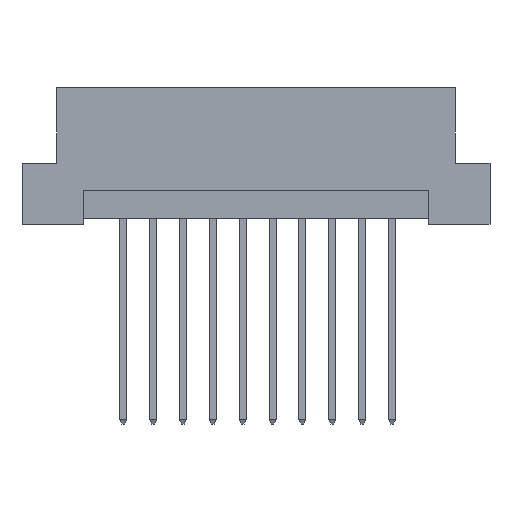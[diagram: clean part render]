
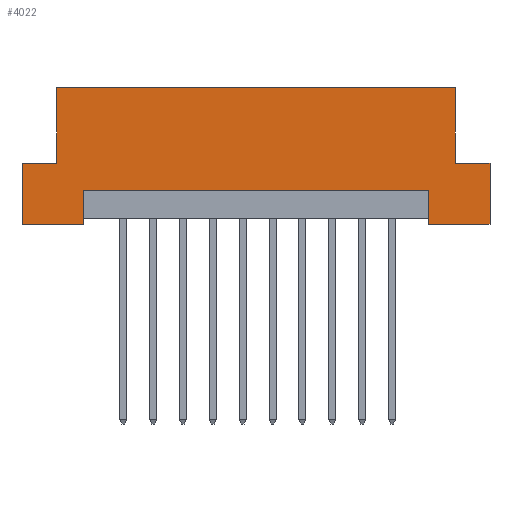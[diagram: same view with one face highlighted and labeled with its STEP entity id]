
A CAD part, front view. The second image highlights one B-rep face of the part: STEP entity #4022.
In plain terms, the highlighted planar face has unit normal (0, -1, 0).
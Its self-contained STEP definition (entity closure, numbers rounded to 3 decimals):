
#50 = CARTESIAN_POINT ( 'NONE',  ( 19.9, 0., 5.2 ) ) ;
#262 = EDGE_LOOP ( 'NONE', ( #6584, #5447, #4503, #2986, #5930, #6435, #2217, #4300, #5325, #4414, #3170, #342 ) ) ;
#336 = LINE ( 'NONE', #4643, #783 ) ;
#342 = ORIENTED_EDGE ( 'NONE', *, *, #4742, .F. ) ;
#356 = PLANE ( 'NONE',  #2508 ) ;
#554 = CARTESIAN_POINT ( 'NONE',  ( -19.9, 0., 5.2 ) ) ;
#592 = CARTESIAN_POINT ( 'NONE',  ( -19.9, 0., 5.2 ) ) ;
#783 = VECTOR ( 'NONE', #5684, 1000. ) ;
#797 = EDGE_CURVE ( 'NONE', #2277, #6769, #2250, .T. ) ;
#870 = CARTESIAN_POINT ( 'NONE',  ( 19.9, 0., 0. ) ) ;
#879 = VECTOR ( 'NONE', #4451, 1000. ) ;
#881 = CARTESIAN_POINT ( 'NONE',  ( -19.9, 0., 0. ) ) ;
#1060 = VECTOR ( 'NONE', #2801, 1000. ) ;
#1104 = EDGE_CURVE ( 'NONE', #5030, #2450, #3329, .T. ) ;
#1120 = LINE ( 'NONE', #592, #4772 ) ;
#1385 = LINE ( 'NONE', #6253, #3183 ) ;
#1445 = CARTESIAN_POINT ( 'NONE',  ( -19.9, 0., 11.6 ) ) ;
#1475 = EDGE_CURVE ( 'NONE', #1818, #4754, #336, .T. ) ;
#1507 = DIRECTION ( 'NONE',  ( 0., 0., 1. ) ) ;
#1660 = LINE ( 'NONE', #5497, #1060 ) ;
#1763 = VERTEX_POINT ( 'NONE', #6901 ) ;
#1818 = VERTEX_POINT ( 'NONE', #3364 ) ;
#1860 = VECTOR ( 'NONE', #6773, 1000. ) ;
#1890 = CARTESIAN_POINT ( 'NONE',  ( -19.9, 0., 0. ) ) ;
#1901 = CARTESIAN_POINT ( 'NONE',  ( -14.69, 0., 0.5 ) ) ;
#2171 = VERTEX_POINT ( 'NONE', #6325 ) ;
#2204 = DIRECTION ( 'NONE',  ( 1., 0., 0. ) ) ;
#2215 = CARTESIAN_POINT ( 'NONE',  ( 14.69, 0., 2.9 ) ) ;
#2217 = ORIENTED_EDGE ( 'NONE', *, *, #1475, .F. ) ;
#2250 = LINE ( 'NONE', #2215, #2349 ) ;
#2277 = VERTEX_POINT ( 'NONE', #3214 ) ;
#2349 = VECTOR ( 'NONE', #5944, 1000. ) ;
#2450 = VERTEX_POINT ( 'NONE', #2934 ) ;
#2483 = EDGE_CURVE ( 'NONE', #2450, #6653, #4736, .T. ) ;
#2508 = AXIS2_PLACEMENT_3D ( 'NONE', #1445, #6988, #1507 ) ;
#2801 = DIRECTION ( 'NONE',  ( 0., 0., 1. ) ) ;
#2822 = EDGE_CURVE ( 'NONE', #2171, #1818, #5633, .T. ) ;
#2891 = LINE ( 'NONE', #1901, #1860 ) ;
#2904 = LINE ( 'NONE', #3502, #5082 ) ;
#2934 = CARTESIAN_POINT ( 'NONE',  ( 19.9, 0., 5.2 ) ) ;
#2986 = ORIENTED_EDGE ( 'NONE', *, *, #2483, .F. ) ;
#3008 = LINE ( 'NONE', #881, #6838 ) ;
#3039 = DIRECTION ( 'NONE',  ( -1., 0., 0. ) ) ;
#3167 = DIRECTION ( 'NONE',  ( 0., 0., -1. ) ) ;
#3170 = ORIENTED_EDGE ( 'NONE', *, *, #3307, .F. ) ;
#3175 = CARTESIAN_POINT ( 'NONE',  ( -14.69, 0., 2.9 ) ) ;
#3183 = VECTOR ( 'NONE', #5683, 1000. ) ;
#3214 = CARTESIAN_POINT ( 'NONE',  ( 14.69, 0., 2.9 ) ) ;
#3263 = VERTEX_POINT ( 'NONE', #1890 ) ;
#3307 = EDGE_CURVE ( 'NONE', #4522, #3263, #1385, .T. ) ;
#3326 = EDGE_CURVE ( 'NONE', #6653, #1763, #3008, .T. ) ;
#3329 = LINE ( 'NONE', #50, #5870 ) ;
#3364 = CARTESIAN_POINT ( 'NONE',  ( -16.94, 0., 11.6 ) ) ;
#3483 = VECTOR ( 'NONE', #3167, 1000. ) ;
#3502 = CARTESIAN_POINT ( 'NONE',  ( 16.94, 0., 5.2 ) ) ;
#3712 = EDGE_CURVE ( 'NONE', #3263, #4529, #1660, .T. ) ;
#3883 = LINE ( 'NONE', #5023, #5916 ) ;
#3956 = DIRECTION ( 'NONE',  ( 0., 0., 1. ) ) ;
#4022 = ADVANCED_FACE ( 'NONE', ( #5272 ), #356, .F. ) ;
#4300 = ORIENTED_EDGE ( 'NONE', *, *, #2822, .F. ) ;
#4414 = ORIENTED_EDGE ( 'NONE', *, *, #3712, .F. ) ;
#4442 = CARTESIAN_POINT ( 'NONE',  ( 16.94, 0., 11.6 ) ) ;
#4451 = DIRECTION ( 'NONE',  ( 0., 0., 1. ) ) ;
#4503 = ORIENTED_EDGE ( 'NONE', *, *, #3326, .F. ) ;
#4522 = VERTEX_POINT ( 'NONE', #6567 ) ;
#4529 = VERTEX_POINT ( 'NONE', #554 ) ;
#4643 = CARTESIAN_POINT ( 'NONE',  ( -19.9, 0., 11.6 ) ) ;
#4705 = CARTESIAN_POINT ( 'NONE',  ( 19.9, 0., 0. ) ) ;
#4736 = LINE ( 'NONE', #870, #3483 ) ;
#4742 = EDGE_CURVE ( 'NONE', #6769, #4522, #2891, .T. ) ;
#4754 = VERTEX_POINT ( 'NONE', #4442 ) ;
#4772 = VECTOR ( 'NONE', #4921, 1000. ) ;
#4921 = DIRECTION ( 'NONE',  ( 1., 0., 0. ) ) ;
#5023 = CARTESIAN_POINT ( 'NONE',  ( 14.69, 0., 0.5 ) ) ;
#5030 = VERTEX_POINT ( 'NONE', #6978 ) ;
#5082 = VECTOR ( 'NONE', #3956, 1000. ) ;
#5251 = EDGE_CURVE ( 'NONE', #5030, #4754, #2904, .T. ) ;
#5272 = FACE_OUTER_BOUND ( 'NONE', #262, .T. ) ;
#5325 = ORIENTED_EDGE ( 'NONE', *, *, #6050, .F. ) ;
#5447 = ORIENTED_EDGE ( 'NONE', *, *, #5958, .T. ) ;
#5497 = CARTESIAN_POINT ( 'NONE',  ( -19.9, 0., 0. ) ) ;
#5633 = LINE ( 'NONE', #6172, #879 ) ;
#5683 = DIRECTION ( 'NONE',  ( -1., 0., 0. ) ) ;
#5684 = DIRECTION ( 'NONE',  ( 1., 0., 0. ) ) ;
#5870 = VECTOR ( 'NONE', #2204, 1000. ) ;
#5916 = VECTOR ( 'NONE', #6673, 1000. ) ;
#5930 = ORIENTED_EDGE ( 'NONE', *, *, #1104, .F. ) ;
#5944 = DIRECTION ( 'NONE',  ( -1., 0., 0. ) ) ;
#5958 = EDGE_CURVE ( 'NONE', #2277, #1763, #3883, .T. ) ;
#6050 = EDGE_CURVE ( 'NONE', #4529, #2171, #1120, .T. ) ;
#6172 = CARTESIAN_POINT ( 'NONE',  ( -16.94, 0., 5.2 ) ) ;
#6253 = CARTESIAN_POINT ( 'NONE',  ( -19.9, 0., 0. ) ) ;
#6325 = CARTESIAN_POINT ( 'NONE',  ( -16.94, 0., 5.2 ) ) ;
#6435 = ORIENTED_EDGE ( 'NONE', *, *, #5251, .T. ) ;
#6567 = CARTESIAN_POINT ( 'NONE',  ( -14.69, 0., 0. ) ) ;
#6584 = ORIENTED_EDGE ( 'NONE', *, *, #797, .F. ) ;
#6653 = VERTEX_POINT ( 'NONE', #4705 ) ;
#6673 = DIRECTION ( 'NONE',  ( 0., 0., -1. ) ) ;
#6769 = VERTEX_POINT ( 'NONE', #3175 ) ;
#6773 = DIRECTION ( 'NONE',  ( 0., 0., -1. ) ) ;
#6838 = VECTOR ( 'NONE', #3039, 1000. ) ;
#6901 = CARTESIAN_POINT ( 'NONE',  ( 14.69, 0., 0. ) ) ;
#6978 = CARTESIAN_POINT ( 'NONE',  ( 16.94, 0., 5.2 ) ) ;
#6988 = DIRECTION ( 'NONE',  ( 0., 1., 0. ) ) ;
